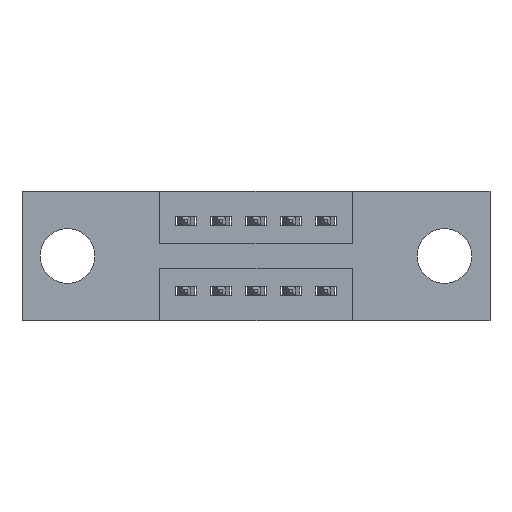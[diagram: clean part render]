
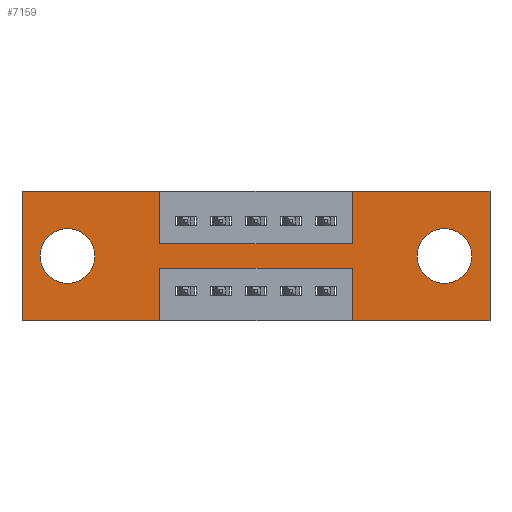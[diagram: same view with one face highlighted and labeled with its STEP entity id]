
A CAD part, front view. The second image highlights one B-rep face of the part: STEP entity #7159.
In plain terms, the highlighted planar face has unit normal (0, -1, 0).
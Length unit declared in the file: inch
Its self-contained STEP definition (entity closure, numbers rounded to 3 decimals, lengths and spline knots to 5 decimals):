
#2 = CARTESIAN_POINT ( 'NONE',  ( 1.335, 0., 0. ) ) ;
#106 = DIRECTION ( 'NONE',  ( 0., 0., -1. ) ) ;
#195 = VECTOR ( 'NONE', #3533, 39.37008 ) ;
#207 = ORIENTED_EDGE ( 'NONE', *, *, #2784, .F. ) ;
#220 = CARTESIAN_POINT ( 'NONE',  ( 0.9425, 0., -0.22 ) ) ;
#254 = LINE ( 'NONE', #4689, #3577 ) ;
#271 = EDGE_CURVE ( 'NONE', #8145, #5103, #254, .T. ) ;
#281 = ORIENTED_EDGE ( 'NONE', *, *, #6869, .F. ) ;
#690 = CARTESIAN_POINT ( 'NONE',  ( 0.9425, 0., -0.37 ) ) ;
#801 = ORIENTED_EDGE ( 'NONE', *, *, #8300, .F. ) ;
#803 = LINE ( 'NONE', #4248, #6728 ) ;
#808 = ORIENTED_EDGE ( 'NONE', *, *, #7223, .F. ) ;
#929 = CARTESIAN_POINT ( 'NONE',  ( 1.205, 0., -0.263 ) ) ;
#962 = EDGE_LOOP ( 'NONE', ( #5593, #5361 ) ) ;
#1129 = VERTEX_POINT ( 'NONE', #690 ) ;
#1256 = CARTESIAN_POINT ( 'NONE',  ( 0., 0., 0. ) ) ;
#1410 = LINE ( 'NONE', #1256, #1652 ) ;
#1415 = DIRECTION ( 'NONE',  ( 0., 0., -1. ) ) ;
#1533 = CARTESIAN_POINT ( 'NONE',  ( 0.3925, 0., -0.15 ) ) ;
#1621 = LINE ( 'NONE', #2, #5201 ) ;
#1652 = VECTOR ( 'NONE', #6253, 39.37008 ) ;
#1775 = VECTOR ( 'NONE', #5406, 39.37008 ) ;
#1779 = DIRECTION ( 'NONE',  ( -1., 0., 0. ) ) ;
#2037 = DIRECTION ( 'NONE',  ( 0., 1., 0. ) ) ;
#2042 = VERTEX_POINT ( 'NONE', #4997 ) ;
#2043 = FACE_BOUND ( 'NONE', #962, .T. ) ;
#2044 = CARTESIAN_POINT ( 'NONE',  ( 1.335, 0., -0.37 ) ) ;
#2072 = VERTEX_POINT ( 'NONE', #3983 ) ;
#2085 = EDGE_CURVE ( 'NONE', #6499, #7357, #7751, .T. ) ;
#2102 = PLANE ( 'NONE',  #4267 ) ;
#2187 = EDGE_CURVE ( 'NONE', #7357, #6499, #8040, .T. ) ;
#2223 = VERTEX_POINT ( 'NONE', #3281 ) ;
#2300 = VECTOR ( 'NONE', #5099, 39.37008 ) ;
#2316 = LINE ( 'NONE', #8819, #7321 ) ;
#2408 = CARTESIAN_POINT ( 'NONE',  ( 0., 0., 0. ) ) ;
#2568 = VECTOR ( 'NONE', #3587, 39.37008 ) ;
#2667 = DIRECTION ( 'NONE',  ( 0., 1., 0. ) ) ;
#2730 = DIRECTION ( 'NONE',  ( 0., 0., 1. ) ) ;
#2743 = EDGE_CURVE ( 'NONE', #3188, #2223, #8131, .T. ) ;
#2784 = EDGE_CURVE ( 'NONE', #8119, #5820, #3970, .T. ) ;
#2791 = LINE ( 'NONE', #5774, #2568 ) ;
#2792 = DIRECTION ( 'NONE',  ( 0., 0., -1. ) ) ;
#2812 = EDGE_CURVE ( 'NONE', #2072, #3243, #2316, .T. ) ;
#2822 = EDGE_CURVE ( 'NONE', #6026, #3443, #8927, .T. ) ;
#2858 = CARTESIAN_POINT ( 'NONE',  ( 1.205, 0., -0.107 ) ) ;
#2952 = EDGE_LOOP ( 'NONE', ( #8661, #801, #808, #281, #5408, #5641, #8306, #207, #5157, #5512, #4412, #7581 ) ) ;
#3005 = DIRECTION ( 'NONE',  ( 0., 1., 0. ) ) ;
#3062 = CARTESIAN_POINT ( 'NONE',  ( 1.205, 0., -0.185 ) ) ;
#3188 = VERTEX_POINT ( 'NONE', #8425 ) ;
#3189 = CARTESIAN_POINT ( 'NONE',  ( 1.205, 0., -0.185 ) ) ;
#3243 = VERTEX_POINT ( 'NONE', #6435 ) ;
#3281 = CARTESIAN_POINT ( 'NONE',  ( 0.13, 0., -0.107 ) ) ;
#3306 = ORIENTED_EDGE ( 'NONE', *, *, #2187, .T. ) ;
#3342 = EDGE_CURVE ( 'NONE', #2042, #2072, #7197, .T. ) ;
#3443 = VERTEX_POINT ( 'NONE', #8058 ) ;
#3446 = FACE_OUTER_BOUND ( 'NONE', #2952, .T. ) ;
#3533 = DIRECTION ( 'NONE',  ( 1., 0., 0. ) ) ;
#3561 = EDGE_CURVE ( 'NONE', #3443, #8119, #8916, .T. ) ;
#3577 = VECTOR ( 'NONE', #8411, 39.37008 ) ;
#3587 = DIRECTION ( 'NONE',  ( 0., 0., 1. ) ) ;
#3618 = EDGE_CURVE ( 'NONE', #3243, #6026, #1410, .T. ) ;
#3714 = CARTESIAN_POINT ( 'NONE',  ( 0.3925, 0., -0.37 ) ) ;
#3731 = DIRECTION ( 'NONE',  ( 0., 1., 0. ) ) ;
#3783 = CARTESIAN_POINT ( 'NONE',  ( 0.3925, 0., 0. ) ) ;
#3917 = CIRCLE ( 'NONE', #5791, 0.078 ) ;
#3970 = LINE ( 'NONE', #1533, #195 ) ;
#3978 = DIRECTION ( 'NONE',  ( 0., 0., -1. ) ) ;
#3983 = CARTESIAN_POINT ( 'NONE',  ( 0.3925, 0., -0.37 ) ) ;
#4054 = AXIS2_PLACEMENT_3D ( 'NONE', #3189, #2037, #3978 ) ;
#4076 = DIRECTION ( 'NONE',  ( -1., 0., 0. ) ) ;
#4248 = CARTESIAN_POINT ( 'NONE',  ( 0.9425, 0., 0. ) ) ;
#4267 = AXIS2_PLACEMENT_3D ( 'NONE', #6374, #7070, #2792 ) ;
#4412 = ORIENTED_EDGE ( 'NONE', *, *, #3618, .F. ) ;
#4604 = EDGE_LOOP ( 'NONE', ( #4831, #3306 ) ) ;
#4689 = CARTESIAN_POINT ( 'NONE',  ( 0., 0., 0. ) ) ;
#4831 = ORIENTED_EDGE ( 'NONE', *, *, #2085, .T. ) ;
#4889 = VERTEX_POINT ( 'NONE', #2044 ) ;
#4987 = EDGE_CURVE ( 'NONE', #5103, #4889, #1621, .T. ) ;
#4988 = DIRECTION ( 'NONE',  ( 0., 0., 1. ) ) ;
#4997 = CARTESIAN_POINT ( 'NONE',  ( 0.3925, 0., -0.22 ) ) ;
#5043 = VECTOR ( 'NONE', #4076, 39.37008 ) ;
#5099 = DIRECTION ( 'NONE',  ( 0., 0., -1. ) ) ;
#5103 = VERTEX_POINT ( 'NONE', #8012 ) ;
#5157 = ORIENTED_EDGE ( 'NONE', *, *, #3561, .F. ) ;
#5201 = VECTOR ( 'NONE', #106, 39.37008 ) ;
#5297 = CARTESIAN_POINT ( 'NONE',  ( 0., 0., -0.37 ) ) ;
#5361 = ORIENTED_EDGE ( 'NONE', *, *, #2743, .T. ) ;
#5406 = DIRECTION ( 'NONE',  ( 0., 0., -1. ) ) ;
#5408 = ORIENTED_EDGE ( 'NONE', *, *, #4987, .F. ) ;
#5512 = ORIENTED_EDGE ( 'NONE', *, *, #2822, .F. ) ;
#5593 = ORIENTED_EDGE ( 'NONE', *, *, #5865, .T. ) ;
#5641 = ORIENTED_EDGE ( 'NONE', *, *, #271, .F. ) ;
#5755 = VECTOR ( 'NONE', #1779, 39.37008 ) ;
#5774 = CARTESIAN_POINT ( 'NONE',  ( 0.9425, 0., -0.37 ) ) ;
#5791 = AXIS2_PLACEMENT_3D ( 'NONE', #7944, #3731, #8530 ) ;
#5820 = VERTEX_POINT ( 'NONE', #6578 ) ;
#5865 = EDGE_CURVE ( 'NONE', #2223, #3188, #3917, .T. ) ;
#6026 = VERTEX_POINT ( 'NONE', #2408 ) ;
#6116 = AXIS2_PLACEMENT_3D ( 'NONE', #8641, #2667, #2730 ) ;
#6169 = CARTESIAN_POINT ( 'NONE',  ( 0.3925, 0., -0.15 ) ) ;
#6216 = CARTESIAN_POINT ( 'NONE',  ( 0.3925, 0., -0.22 ) ) ;
#6253 = DIRECTION ( 'NONE',  ( 0., 0., 1. ) ) ;
#6374 = CARTESIAN_POINT ( 'NONE',  ( 0., 0., -0.37 ) ) ;
#6435 = CARTESIAN_POINT ( 'NONE',  ( 0., 0., -0.37 ) ) ;
#6440 = EDGE_CURVE ( 'NONE', #5820, #8145, #803, .T. ) ;
#6499 = VERTEX_POINT ( 'NONE', #2858 ) ;
#6578 = CARTESIAN_POINT ( 'NONE',  ( 0.9425, 0., -0.15 ) ) ;
#6728 = VECTOR ( 'NONE', #4988, 39.37008 ) ;
#6793 = VERTEX_POINT ( 'NONE', #220 ) ;
#6869 = EDGE_CURVE ( 'NONE', #4889, #1129, #7603, .T. ) ;
#7070 = DIRECTION ( 'NONE',  ( 0., -1., 0. ) ) ;
#7159 = ADVANCED_FACE ( 'NONE', ( #8690, #2043, #3446 ), #2102, .T. ) ;
#7197 = LINE ( 'NONE', #3714, #1775 ) ;
#7223 = EDGE_CURVE ( 'NONE', #1129, #6793, #2791, .T. ) ;
#7231 = CARTESIAN_POINT ( 'NONE',  ( 0., 0., 0. ) ) ;
#7321 = VECTOR ( 'NONE', #7926, 39.37008 ) ;
#7357 = VERTEX_POINT ( 'NONE', #929 ) ;
#7581 = ORIENTED_EDGE ( 'NONE', *, *, #2812, .F. ) ;
#7603 = LINE ( 'NONE', #5297, #5755 ) ;
#7751 = CIRCLE ( 'NONE', #4054, 0.078 ) ;
#7830 = AXIS2_PLACEMENT_3D ( 'NONE', #3062, #3005, #1415 ) ;
#7926 = DIRECTION ( 'NONE',  ( -1., 0., 0. ) ) ;
#7928 = DIRECTION ( 'NONE',  ( 1., 0., 0. ) ) ;
#7944 = CARTESIAN_POINT ( 'NONE',  ( 0.13, 0., -0.185 ) ) ;
#8012 = CARTESIAN_POINT ( 'NONE',  ( 1.335, 0., 0. ) ) ;
#8040 = CIRCLE ( 'NONE', #7830, 0.078 ) ;
#8058 = CARTESIAN_POINT ( 'NONE',  ( 0.3925, 0., 0. ) ) ;
#8119 = VERTEX_POINT ( 'NONE', #6169 ) ;
#8131 = CIRCLE ( 'NONE', #6116, 0.078 ) ;
#8145 = VERTEX_POINT ( 'NONE', #8188 ) ;
#8188 = CARTESIAN_POINT ( 'NONE',  ( 0.9425, 0., 0. ) ) ;
#8300 = EDGE_CURVE ( 'NONE', #6793, #2042, #8577, .T. ) ;
#8306 = ORIENTED_EDGE ( 'NONE', *, *, #6440, .F. ) ;
#8411 = DIRECTION ( 'NONE',  ( 1., 0., 0. ) ) ;
#8425 = CARTESIAN_POINT ( 'NONE',  ( 0.13, 0., -0.263 ) ) ;
#8530 = DIRECTION ( 'NONE',  ( 0., 0., 1. ) ) ;
#8577 = LINE ( 'NONE', #6216, #5043 ) ;
#8641 = CARTESIAN_POINT ( 'NONE',  ( 0.13, 0., -0.185 ) ) ;
#8661 = ORIENTED_EDGE ( 'NONE', *, *, #3342, .F. ) ;
#8690 = FACE_BOUND ( 'NONE', #4604, .T. ) ;
#8743 = VECTOR ( 'NONE', #7928, 39.37008 ) ;
#8819 = CARTESIAN_POINT ( 'NONE',  ( 0., 0., -0.37 ) ) ;
#8916 = LINE ( 'NONE', #3783, #2300 ) ;
#8927 = LINE ( 'NONE', #7231, #8743 ) ;
